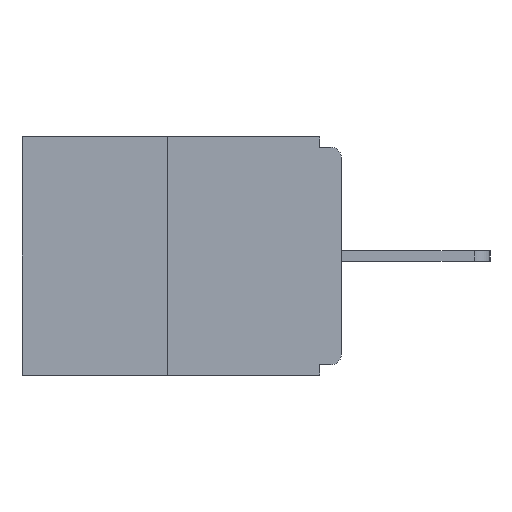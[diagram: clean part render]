
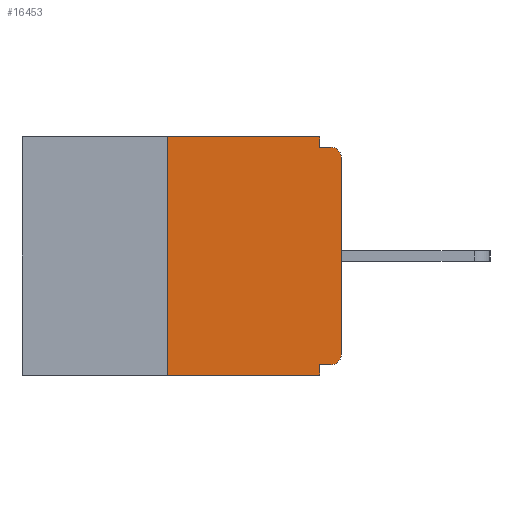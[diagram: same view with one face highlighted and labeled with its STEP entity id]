
A CAD part, left-side view. The second image highlights one B-rep face of the part: STEP entity #16453.
In plain terms, the highlighted planar face has unit normal (-1, 0, 0).
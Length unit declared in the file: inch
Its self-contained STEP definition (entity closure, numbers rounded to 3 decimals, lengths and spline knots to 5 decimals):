
#74 = VERTEX_POINT ( 'NONE', #22397 ) ;
#636 = EDGE_CURVE ( 'NONE', #12092, #5202, #13419, .T. ) ;
#777 = VECTOR ( 'NONE', #3765, 39.37008 ) ;
#1559 = DIRECTION ( 'NONE',  ( 0., 0., -1. ) ) ;
#1670 = VECTOR ( 'NONE', #21128, 39.37008 ) ;
#1737 = VECTOR ( 'NONE', #12433, 39.37008 ) ;
#2515 = CIRCLE ( 'NONE', #9488, 0.015 ) ;
#2572 = AXIS2_PLACEMENT_3D ( 'NONE', #11136, #24629, #13103 ) ;
#2680 = VERTEX_POINT ( 'NONE', #20026 ) ;
#2816 = VECTOR ( 'NONE', #20764, 39.37008 ) ;
#2882 = DIRECTION ( 'NONE',  ( 0., 0., 1. ) ) ;
#2888 = VERTEX_POINT ( 'NONE', #22154 ) ;
#2994 = VECTOR ( 'NONE', #19856, 39.37008 ) ;
#3044 = CIRCLE ( 'NONE', #4353, 0.015 ) ;
#3235 = EDGE_CURVE ( 'NONE', #5202, #3861, #5565, .T. ) ;
#3765 = DIRECTION ( 'NONE',  ( 0., -1., 0. ) ) ;
#3861 = VERTEX_POINT ( 'NONE', #22907 ) ;
#4267 = ORIENTED_EDGE ( 'NONE', *, *, #8806, .T. ) ;
#4353 = AXIS2_PLACEMENT_3D ( 'NONE', #25036, #13521, #1559 ) ;
#4450 = CARTESIAN_POINT ( 'NONE',  ( 0., 0., -0.03 ) ) ;
#4669 = VECTOR ( 'NONE', #16890, 39.37008 ) ;
#4751 = EDGE_CURVE ( 'NONE', #2888, #21690, #7016, .T. ) ;
#4799 = DIRECTION ( 'NONE',  ( -1., 0., 0. ) ) ;
#4919 = ORIENTED_EDGE ( 'NONE', *, *, #9984, .F. ) ;
#5202 = VERTEX_POINT ( 'NONE', #18596 ) ;
#5565 = LINE ( 'NONE', #8310, #777 ) ;
#6167 = ORIENTED_EDGE ( 'NONE', *, *, #15717, .T. ) ;
#6779 = ORIENTED_EDGE ( 'NONE', *, *, #636, .F. ) ;
#7016 = LINE ( 'NONE', #23326, #1670 ) ;
#8161 = CARTESIAN_POINT ( 'NONE',  ( 0., 0.031, -0.343 ) ) ;
#8310 = CARTESIAN_POINT ( 'NONE',  ( 0., 0., -0.015 ) ) ;
#8374 = LINE ( 'NONE', #12241, #2994 ) ;
#8700 = VECTOR ( 'NONE', #2882, 39.37008 ) ;
#8806 = EDGE_CURVE ( 'NONE', #74, #21690, #15203, .T. ) ;
#8888 = CARTESIAN_POINT ( 'NONE',  ( 0., 0.25, 0. ) ) ;
#8993 = VERTEX_POINT ( 'NONE', #10513 ) ;
#9009 = ORIENTED_EDGE ( 'NONE', *, *, #18865, .F. ) ;
#9488 = AXIS2_PLACEMENT_3D ( 'NONE', #16623, #4799, #18598 ) ;
#9984 = EDGE_CURVE ( 'NONE', #2680, #2888, #22695, .T. ) ;
#10074 = CARTESIAN_POINT ( 'NONE',  ( 0., 0.031, 0. ) ) ;
#10135 = EDGE_CURVE ( 'NONE', #74, #8993, #19122, .T. ) ;
#10329 = FACE_OUTER_BOUND ( 'NONE', #15161, .T. ) ;
#10436 = CARTESIAN_POINT ( 'NONE',  ( 0., 0., -0.328 ) ) ;
#10513 = CARTESIAN_POINT ( 'NONE',  ( 0., 0.25, 0. ) ) ;
#10859 = ORIENTED_EDGE ( 'NONE', *, *, #20951, .T. ) ;
#11136 = CARTESIAN_POINT ( 'NONE',  ( 0., 0.46, 0. ) ) ;
#12092 = VERTEX_POINT ( 'NONE', #22814 ) ;
#12241 = CARTESIAN_POINT ( 'NONE',  ( 0., 0., 0. ) ) ;
#12433 = DIRECTION ( 'NONE',  ( 0., 1., 0. ) ) ;
#13103 = DIRECTION ( 'NONE',  ( 0., 0., -1. ) ) ;
#13419 = LINE ( 'NONE', #10074, #2816 ) ;
#13521 = DIRECTION ( 'NONE',  ( -1., 0., 0. ) ) ;
#14196 = ORIENTED_EDGE ( 'NONE', *, *, #10135, .F. ) ;
#14662 = VECTOR ( 'NONE', #25434, 39.37008 ) ;
#15161 = EDGE_LOOP ( 'NONE', ( #9009, #14196, #4267, #25032, #4919, #10859, #16055, #6167, #16647, #6779 ) ) ;
#15203 = LINE ( 'NONE', #17892, #4669 ) ;
#15717 = EDGE_CURVE ( 'NONE', #21785, #3861, #2515, .T. ) ;
#16055 = ORIENTED_EDGE ( 'NONE', *, *, #21741, .T. ) ;
#16453 = ADVANCED_FACE ( 'NONE', ( #10329 ), #22747, .F. ) ;
#16623 = CARTESIAN_POINT ( 'NONE',  ( 0., 0.015, -0.03 ) ) ;
#16647 = ORIENTED_EDGE ( 'NONE', *, *, #3235, .F. ) ;
#16890 = DIRECTION ( 'NONE',  ( 0., -1., 0. ) ) ;
#17892 = CARTESIAN_POINT ( 'NONE',  ( 0., 0.46, -0.343 ) ) ;
#18596 = CARTESIAN_POINT ( 'NONE',  ( 0., 0.031, -0.015 ) ) ;
#18598 = DIRECTION ( 'NONE',  ( 0., 0., -1. ) ) ;
#18865 = EDGE_CURVE ( 'NONE', #8993, #12092, #19917, .T. ) ;
#19122 = LINE ( 'NONE', #8888, #8700 ) ;
#19792 = CARTESIAN_POINT ( 'NONE',  ( 0., 0.46, 0. ) ) ;
#19856 = DIRECTION ( 'NONE',  ( 0., 0., 1. ) ) ;
#19887 = CARTESIAN_POINT ( 'NONE',  ( 0., 0., -0.313 ) ) ;
#19917 = LINE ( 'NONE', #19792, #14662 ) ;
#20026 = CARTESIAN_POINT ( 'NONE',  ( 0., 0.015, -0.328 ) ) ;
#20764 = DIRECTION ( 'NONE',  ( 0., 0., -1. ) ) ;
#20951 = EDGE_CURVE ( 'NONE', #2680, #21086, #3044, .T. ) ;
#21086 = VERTEX_POINT ( 'NONE', #19887 ) ;
#21128 = DIRECTION ( 'NONE',  ( 0., 0., -1. ) ) ;
#21690 = VERTEX_POINT ( 'NONE', #8161 ) ;
#21741 = EDGE_CURVE ( 'NONE', #21086, #21785, #8374, .T. ) ;
#21785 = VERTEX_POINT ( 'NONE', #4450 ) ;
#22154 = CARTESIAN_POINT ( 'NONE',  ( 0., 0.031, -0.328 ) ) ;
#22397 = CARTESIAN_POINT ( 'NONE',  ( 0., 0.25, -0.343 ) ) ;
#22695 = LINE ( 'NONE', #10436, #1737 ) ;
#22747 = PLANE ( 'NONE',  #2572 ) ;
#22814 = CARTESIAN_POINT ( 'NONE',  ( 0., 0.031, 0. ) ) ;
#22907 = CARTESIAN_POINT ( 'NONE',  ( 0., 0.015, -0.015 ) ) ;
#23326 = CARTESIAN_POINT ( 'NONE',  ( 0., 0.031, -0.343 ) ) ;
#24629 = DIRECTION ( 'NONE',  ( 1., 0., 0. ) ) ;
#25032 = ORIENTED_EDGE ( 'NONE', *, *, #4751, .F. ) ;
#25036 = CARTESIAN_POINT ( 'NONE',  ( 0., 0.015, -0.313 ) ) ;
#25434 = DIRECTION ( 'NONE',  ( 0., -1., 0. ) ) ;
